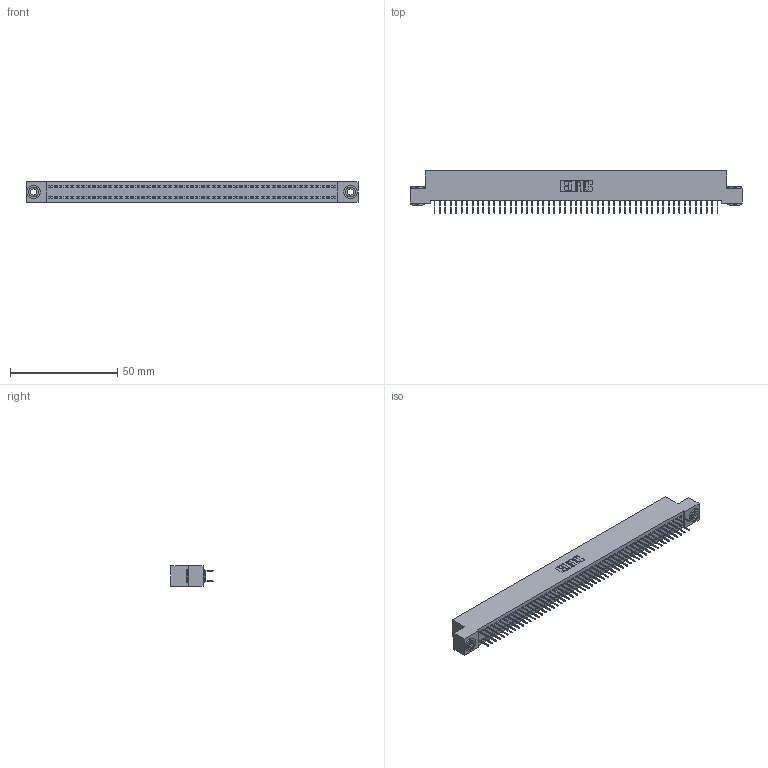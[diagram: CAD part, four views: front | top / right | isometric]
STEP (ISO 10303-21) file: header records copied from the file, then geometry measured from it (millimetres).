
FILE_DESCRIPTION (( 'STEP AP203' ), '1' );
FILE_NAME ('392-106-524-203.STEP', '2019-10-09T22:28:30', ( '' ), ( '' ), 'SwSTEP 2.0', 'SolidWorks 2016', '' );
FILE_SCHEMA (( 'CONFIG_CONTROL_DESIGN' ));
Length unit declared in the file: inch
Products named in the file (4): 342-250-002_345-250-002-102; 392-106-524-203; 342 Part_.156 TH; 345-292-001_345-293-124
Assembly tree (109 placements, depth 2):
  392-106-524-203
    342 Part_.156 TH
    345-292-001_345-293-124  x106
    342-250-002_345-250-002-102  x2
Bounding box: 154.94 x 19.69 x 9.4 mm (x, y, z)
Volume: 13835.8 mm3; surface area: 22589.1 mm2
Topology: 109 solids, 109 shells, 6084 faces, 17229 edges, 11058 vertices
Faces by surface type: plane 4528, cylinder 1548, cone 8
Entity records: 33266 total; most frequent: CARTESIAN_POINT 5473, ORIENTED_EDGE 5402, DIRECTION 4691, EDGE_CURVE 2701, VECTOR 2553, LINE 2553, VERTEX_POINT 1794, AXIS2_PLACEMENT_3D 1069
